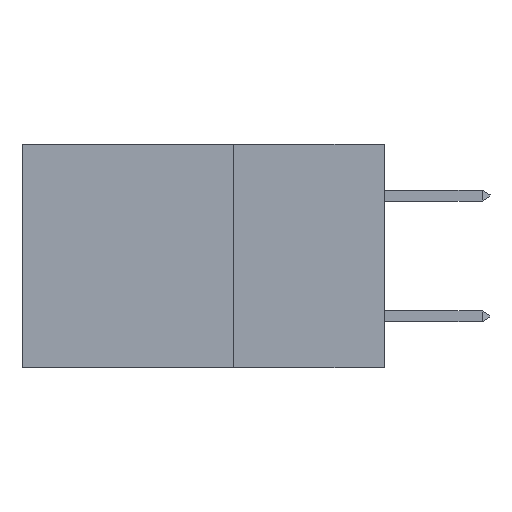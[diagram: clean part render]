
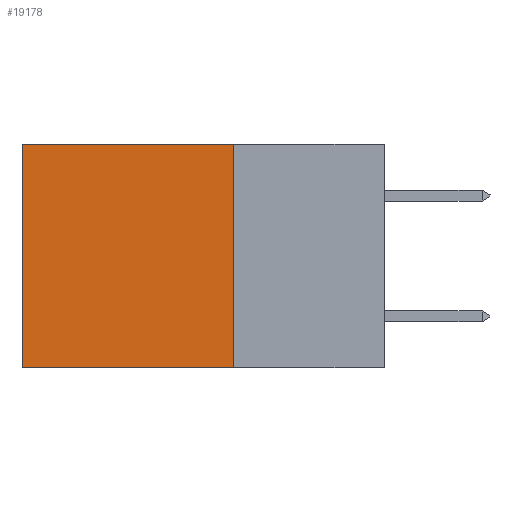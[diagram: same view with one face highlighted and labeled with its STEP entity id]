
A CAD part, left-side view. The second image highlights one B-rep face of the part: STEP entity #19178.
In plain terms, the highlighted planar face has unit normal (-1, 0, 0).
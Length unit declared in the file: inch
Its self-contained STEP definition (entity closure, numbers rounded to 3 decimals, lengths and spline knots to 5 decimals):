
#332 = LINE ( 'NONE', #39293, #37579 ) ;
#751 = VERTEX_POINT ( 'NONE', #28621 ) ;
#965 = VERTEX_POINT ( 'NONE', #37104 ) ;
#5012 = EDGE_LOOP ( 'NONE', ( #35767, #26907, #32351, #7501 ) ) ;
#5744 = EDGE_CURVE ( 'NONE', #751, #7703, #25428, .T. ) ;
#6070 = VECTOR ( 'NONE', #41602, 39.37008 ) ;
#7098 = AXIS2_PLACEMENT_3D ( 'NONE', #7381, #26441, #20187 ) ;
#7381 = CARTESIAN_POINT ( 'NONE',  ( 0.2875, 0.25, 0. ) ) ;
#7501 = ORIENTED_EDGE ( 'NONE', *, *, #5744, .T. ) ;
#7703 = VERTEX_POINT ( 'NONE', #8577 ) ;
#8577 = CARTESIAN_POINT ( 'NONE',  ( 0.2875, 0.6, 0. ) ) ;
#10492 = PLANE ( 'NONE',  #7098 ) ;
#12377 = DIRECTION ( 'NONE',  ( 0., 1., 0. ) ) ;
#15391 = CARTESIAN_POINT ( 'NONE',  ( 0.2875, 0.25, 0. ) ) ;
#19178 = ADVANCED_FACE ( 'NONE', ( #37394 ), #10492, .F. ) ;
#20187 = DIRECTION ( 'NONE',  ( 0., 0., -1. ) ) ;
#21823 = EDGE_CURVE ( 'NONE', #33062, #965, #332, .T. ) ;
#23246 = LINE ( 'NONE', #40251, #40568 ) ;
#23999 = VECTOR ( 'NONE', #36671, 39.37008 ) ;
#25428 = LINE ( 'NONE', #15391, #6070 ) ;
#26006 = LINE ( 'NONE', #39962, #23999 ) ;
#26209 = EDGE_CURVE ( 'NONE', #7703, #965, #26006, .T. ) ;
#26441 = DIRECTION ( 'NONE',  ( 1., 0., 0. ) ) ;
#26907 = ORIENTED_EDGE ( 'NONE', *, *, #21823, .F. ) ;
#27123 = DIRECTION ( 'NONE',  ( 0., 0., -1. ) ) ;
#28621 = CARTESIAN_POINT ( 'NONE',  ( 0.2875, 0.25, 0. ) ) ;
#29308 = CARTESIAN_POINT ( 'NONE',  ( 0.2875, 0.25, -0.37 ) ) ;
#32351 = ORIENTED_EDGE ( 'NONE', *, *, #36866, .F. ) ;
#33062 = VERTEX_POINT ( 'NONE', #29308 ) ;
#35767 = ORIENTED_EDGE ( 'NONE', *, *, #26209, .T. ) ;
#36671 = DIRECTION ( 'NONE',  ( 0., 0., -1. ) ) ;
#36866 = EDGE_CURVE ( 'NONE', #751, #33062, #23246, .T. ) ;
#37104 = CARTESIAN_POINT ( 'NONE',  ( 0.2875, 0.6, -0.37 ) ) ;
#37394 = FACE_OUTER_BOUND ( 'NONE', #5012, .T. ) ;
#37579 = VECTOR ( 'NONE', #12377, 39.37008 ) ;
#39293 = CARTESIAN_POINT ( 'NONE',  ( 0.2875, 0.25, -0.37 ) ) ;
#39962 = CARTESIAN_POINT ( 'NONE',  ( 0.2875, 0.6, 0. ) ) ;
#40251 = CARTESIAN_POINT ( 'NONE',  ( 0.2875, 0.25, 0. ) ) ;
#40568 = VECTOR ( 'NONE', #27123, 39.37008 ) ;
#41602 = DIRECTION ( 'NONE',  ( 0., 1., 0. ) ) ;
